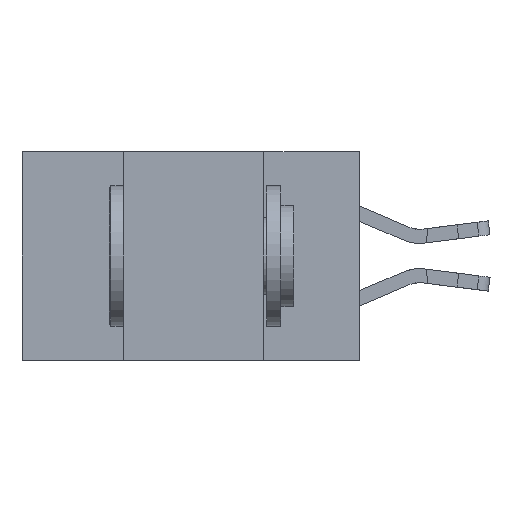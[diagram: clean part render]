
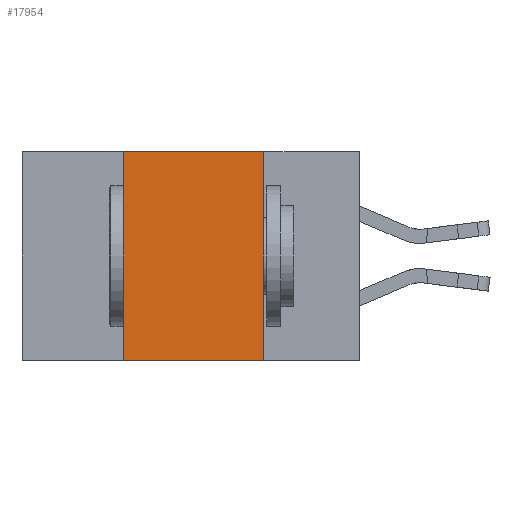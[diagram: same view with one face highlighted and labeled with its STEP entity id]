
A CAD part, left-side view. The second image highlights one B-rep face of the part: STEP entity #17954.
In plain terms, the highlighted planar face has unit normal (-1, 0, 0).
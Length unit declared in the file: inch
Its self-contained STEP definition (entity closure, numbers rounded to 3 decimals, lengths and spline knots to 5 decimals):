
#533 = EDGE_LOOP ( 'NONE', ( #14931, #17591, #14078, #9426 ) ) ;
#1053 = EDGE_CURVE ( 'NONE', #20330, #14219, #6930, .T. ) ;
#2007 = LINE ( 'NONE', #18101, #20260 ) ;
#3403 = CARTESIAN_POINT ( 'NONE',  ( 0., 0.42, -0.37 ) ) ;
#3534 = VERTEX_POINT ( 'NONE', #3403 ) ;
#3854 = CARTESIAN_POINT ( 'NONE',  ( 0., 0.6, 0. ) ) ;
#4512 = VECTOR ( 'NONE', #20532, 39.37008 ) ;
#5736 = DIRECTION ( 'NONE',  ( 0., 0., -1. ) ) ;
#6930 = LINE ( 'NONE', #23029, #15622 ) ;
#7255 = VECTOR ( 'NONE', #19714, 39.37008 ) ;
#9125 = FACE_OUTER_BOUND ( 'NONE', #533, .T. ) ;
#9426 = ORIENTED_EDGE ( 'NONE', *, *, #14231, .T. ) ;
#10055 = CARTESIAN_POINT ( 'NONE',  ( 0., 0.17, -0.37 ) ) ;
#10294 = EDGE_CURVE ( 'NONE', #3534, #17243, #21126, .T. ) ;
#10883 = DIRECTION ( 'NONE',  ( 0., 0., -1. ) ) ;
#12250 = CARTESIAN_POINT ( 'NONE',  ( 0., 0.42, 0. ) ) ;
#13901 = AXIS2_PLACEMENT_3D ( 'NONE', #3854, #16154, #5736 ) ;
#14078 = ORIENTED_EDGE ( 'NONE', *, *, #10294, .F. ) ;
#14219 = VERTEX_POINT ( 'NONE', #10055 ) ;
#14231 = EDGE_CURVE ( 'NONE', #3534, #14219, #22056, .T. ) ;
#14931 = ORIENTED_EDGE ( 'NONE', *, *, #1053, .F. ) ;
#15622 = VECTOR ( 'NONE', #10883, 39.37008 ) ;
#16154 = DIRECTION ( 'NONE',  ( 1., 0., 0. ) ) ;
#16443 = DIRECTION ( 'NONE',  ( 0., -1., 0. ) ) ;
#17243 = VERTEX_POINT ( 'NONE', #12250 ) ;
#17591 = ORIENTED_EDGE ( 'NONE', *, *, #18081, .F. ) ;
#17954 = ADVANCED_FACE ( 'NONE', ( #9125 ), #21363, .F. ) ;
#18081 = EDGE_CURVE ( 'NONE', #17243, #20330, #2007, .T. ) ;
#18101 = CARTESIAN_POINT ( 'NONE',  ( 0., 0.6, 0. ) ) ;
#18758 = CARTESIAN_POINT ( 'NONE',  ( 0., 0.6, -0.37 ) ) ;
#19714 = DIRECTION ( 'NONE',  ( 0., 0., 1. ) ) ;
#20260 = VECTOR ( 'NONE', #16443, 39.37008 ) ;
#20330 = VERTEX_POINT ( 'NONE', #21697 ) ;
#20532 = DIRECTION ( 'NONE',  ( 0., -1., 0. ) ) ;
#21126 = LINE ( 'NONE', #21410, #7255 ) ;
#21363 = PLANE ( 'NONE',  #13901 ) ;
#21410 = CARTESIAN_POINT ( 'NONE',  ( 0., 0.42, 0. ) ) ;
#21697 = CARTESIAN_POINT ( 'NONE',  ( 0., 0.17, 0. ) ) ;
#22056 = LINE ( 'NONE', #18758, #4512 ) ;
#23029 = CARTESIAN_POINT ( 'NONE',  ( 0., 0.17, 0. ) ) ;
